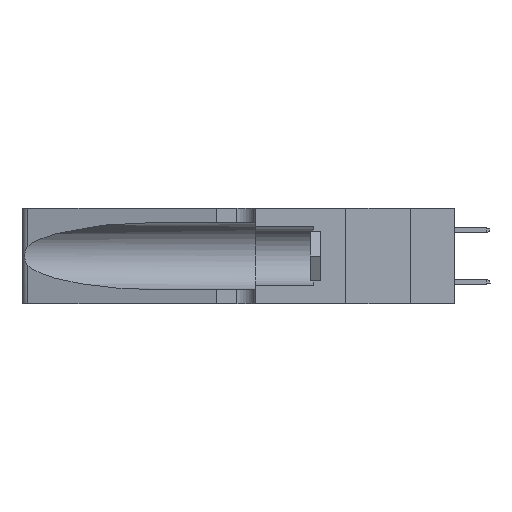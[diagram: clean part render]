
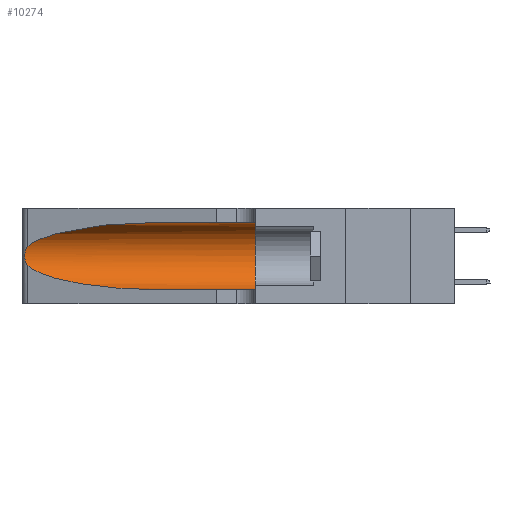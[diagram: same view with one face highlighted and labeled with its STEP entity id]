
A CAD part, left-side view. The second image highlights one B-rep face of the part: STEP entity #10274.
In plain terms, the highlighted cylindrical face has radius 3.308 mm (diameter 6.617 mm), a partial arc.
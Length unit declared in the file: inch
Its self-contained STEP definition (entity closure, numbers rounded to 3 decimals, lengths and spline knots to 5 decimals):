
#402 = EDGE_CURVE ( 'NONE', #16344, #21467, #15024, .T. ) ;
#472 = CARTESIAN_POINT ( 'NONE',  ( 0.1305, 0.35, 0.31525 ) ) ;
#1538 = LINE ( 'NONE', #10030, #15409 ) ;
#1576 = DIRECTION ( 'NONE',  ( 0., 1., 0. ) ) ;
#2513 = CARTESIAN_POINT ( 'NONE',  ( 0.25854, 1.2359, 0.20912 ) ) ;
#2620 = CARTESIAN_POINT ( 'NONE',  ( 0.25487, 1.22718, 0.22369 ) ) ;
#2865 = VERTEX_POINT ( 'NONE', #8255 ) ;
#2905 = CARTESIAN_POINT ( 'NONE',  ( 0.25487, 1.22718, 0.22369 ) ) ;
#3159 = ORIENTED_EDGE ( 'NONE', *, *, #10914, .F. ) ;
#3823 = CARTESIAN_POINT ( 'NONE',  ( 0.25487, 1.22718, 0.22369 ) ) ;
#3981 = DIRECTION ( 'NONE',  ( 0., -1., 0. ) ) ;
#4791 = CARTESIAN_POINT ( 'NONE',  ( 0.25555, 1.22994, 0.2215 ) ) ;
#5371 = CARTESIAN_POINT ( 'NONE',  ( 0.2373, 1.15595, 0.08982 ) ) ;
#5971 = DIRECTION ( 'NONE',  ( 0., 0., -1. ) ) ;
#5999 = ORIENTED_EDGE ( 'NONE', *, *, #402, .T. ) ;
#6860 = AXIS2_PLACEMENT_3D ( 'NONE', #19747, #1576, #9678 ) ;
#6913 = CARTESIAN_POINT ( 'NONE',  ( 0.26018, 1.23835, 0.19895 ) ) ;
#7025 = EDGE_CURVE ( 'NONE', #13130, #2865, #17049, .T. ) ;
#7475 = EDGE_LOOP ( 'NONE', ( #23087, #18155, #19377, #5999, #3159, #24619 ) ) ;
#7818 = CARTESIAN_POINT ( 'NONE',  ( 0.1305, 0.72297, 0.31525 ) ) ;
#8255 = CARTESIAN_POINT ( 'NONE',  ( 0.25487, 1.22718, 0.14631 ) ) ;
#8889 = VECTOR ( 'NONE', #13307, 39.37008 ) ;
#9040 = CARTESIAN_POINT ( 'NONE',  ( 0.25639, 1.23186, 0.15144 ) ) ;
#9172 = CARTESIAN_POINT ( 'NONE',  ( 0.25787, 1.23484, 0.2124 ) ) ;
#9678 = DIRECTION ( 'NONE',  ( 0., 0., 1. ) ) ;
#9960 = FACE_OUTER_BOUND ( 'NONE', #7475, .T. ) ;
#10030 = CARTESIAN_POINT ( 'NONE',  ( 0.1305, 1.61858, 0.31525 ) ) ;
#10096 = CARTESIAN_POINT ( 'NONE',  ( 0.1305, 0.35, 0.05475 ) ) ;
#10274 = ADVANCED_FACE ( 'NONE', ( #9960 ), #20156, .F. ) ;
#10914 = EDGE_CURVE ( 'NONE', #25817, #21467, #23784, .T. ) ;
#13130 = VERTEX_POINT ( 'NONE', #2620 ) ;
#13307 = DIRECTION ( 'NONE',  ( 0., -1., 0. ) ) ;
#13637 = EDGE_CURVE ( 'NONE', #2865, #16344, #13657, .T. ) ;
#13657 =( BOUNDED_CURVE ( )  B_SPLINE_CURVE ( 3, ( #23660, #5371, #17671, #17273 ),
 .UNSPECIFIED., .F., .T. ) 
 B_SPLINE_CURVE_WITH_KNOTS ( ( 4, 4 ),
 ( 3.44316, 4.71239 ),
 .UNSPECIFIED. ) 
 CURVE ( )  GEOMETRIC_REPRESENTATION_ITEM ( )  RATIONAL_B_SPLINE_CURVE ( ( 1., 0.87, 0.87, 1. ) ) 
 REPRESENTATION_ITEM ( '' )  );
#14254 = DIRECTION ( 'NONE',  ( 0., -1., 0. ) ) ;
#14255 = EDGE_CURVE ( 'NONE', #18482, #25817, #1538, .T. ) ;
#14496 =( BOUNDED_CURVE ( )  B_SPLINE_CURVE ( 3, ( #7818, #15884, #23982, #3823 ),
 .UNSPECIFIED., .F., .F. ) 
 B_SPLINE_CURVE_WITH_KNOTS ( ( 4, 4 ),
 ( 1.5708, 2.84003 ),
 .UNSPECIFIED. ) 
 CURVE ( )  GEOMETRIC_REPRESENTATION_ITEM ( )  RATIONAL_B_SPLINE_CURVE ( ( 1., 0.87, 0.87, 1. ) ) 
 REPRESENTATION_ITEM ( '' )  );
#14989 = CARTESIAN_POINT ( 'NONE',  ( 0.26075, 1.23896, 0.19203 ) ) ;
#15024 = LINE ( 'NONE', #17387, #8889 ) ;
#15409 = VECTOR ( 'NONE', #14254, 39.37008 ) ;
#15884 = CARTESIAN_POINT ( 'NONE',  ( 0.18966, 0.96281, 0.31525 ) ) ;
#16344 = VERTEX_POINT ( 'NONE', #20586 ) ;
#17049 = B_SPLINE_CURVE_WITH_KNOTS ( 'NONE', 3,
 ( #2905, #4791, #20675, #9172, #2513, #6913, #14989, #17214, #24925, #23092, #23216, #9040, #19222, #18838 ),
 .UNSPECIFIED., .F., .F.,
 ( 4, 2, 2, 2, 2, 2, 4 ),
 ( 0., 0.00027, 0.00053, 0.00107, 0.0016, 0.00187, 0.00214 ),
 .UNSPECIFIED. ) ;
#17214 = CARTESIAN_POINT ( 'NONE',  ( 0.26075, 1.23896, 0.178 ) ) ;
#17273 = CARTESIAN_POINT ( 'NONE',  ( 0.1305, 0.72297, 0.05475 ) ) ;
#17387 = CARTESIAN_POINT ( 'NONE',  ( 0.1305, 1.61858, 0.05475 ) ) ;
#17671 = CARTESIAN_POINT ( 'NONE',  ( 0.18966, 0.96281, 0.05475 ) ) ;
#18155 = ORIENTED_EDGE ( 'NONE', *, *, #7025, .T. ) ;
#18482 = VERTEX_POINT ( 'NONE', #24999 ) ;
#18838 = CARTESIAN_POINT ( 'NONE',  ( 0.25487, 1.22718, 0.14631 ) ) ;
#19222 = CARTESIAN_POINT ( 'NONE',  ( 0.25555, 1.22993, 0.14849 ) ) ;
#19377 = ORIENTED_EDGE ( 'NONE', *, *, #13637, .T. ) ;
#19747 = CARTESIAN_POINT ( 'NONE',  ( 0.1305, 0.35, 0.185 ) ) ;
#20156 = CYLINDRICAL_SURFACE ( 'NONE', #25869, 0.13025 ) ;
#20586 = CARTESIAN_POINT ( 'NONE',  ( 0.1305, 0.72297, 0.05475 ) ) ;
#20675 = CARTESIAN_POINT ( 'NONE',  ( 0.25639, 1.23184, 0.21858 ) ) ;
#21467 = VERTEX_POINT ( 'NONE', #10096 ) ;
#22755 = EDGE_CURVE ( 'NONE', #18482, #13130, #14496, .T. ) ;
#23087 = ORIENTED_EDGE ( 'NONE', *, *, #22755, .T. ) ;
#23092 = CARTESIAN_POINT ( 'NONE',  ( 0.25856, 1.23593, 0.16098 ) ) ;
#23216 = CARTESIAN_POINT ( 'NONE',  ( 0.25789, 1.23486, 0.15765 ) ) ;
#23660 = CARTESIAN_POINT ( 'NONE',  ( 0.25487, 1.22718, 0.14631 ) ) ;
#23784 = CIRCLE ( 'NONE', #6860, 0.13025 ) ;
#23982 = CARTESIAN_POINT ( 'NONE',  ( 0.2373, 1.15595, 0.28018 ) ) ;
#24126 = CARTESIAN_POINT ( 'NONE',  ( 0.1305, 1.61858, 0.185 ) ) ;
#24619 = ORIENTED_EDGE ( 'NONE', *, *, #14255, .F. ) ;
#24925 = CARTESIAN_POINT ( 'NONE',  ( 0.26017, 1.23833, 0.17102 ) ) ;
#24999 = CARTESIAN_POINT ( 'NONE',  ( 0.1305, 0.72297, 0.31525 ) ) ;
#25817 = VERTEX_POINT ( 'NONE', #472 ) ;
#25869 = AXIS2_PLACEMENT_3D ( 'NONE', #24126, #3981, #5971 ) ;
